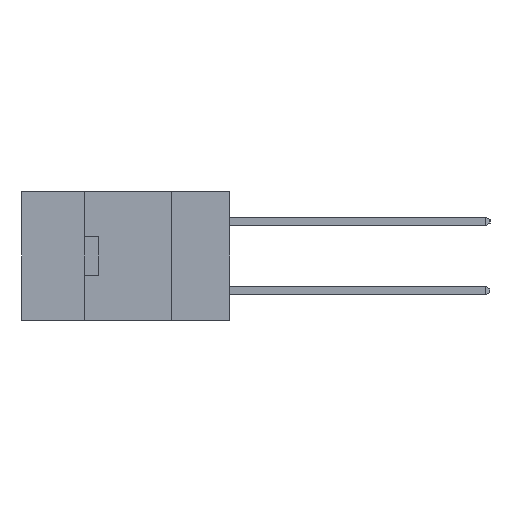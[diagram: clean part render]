
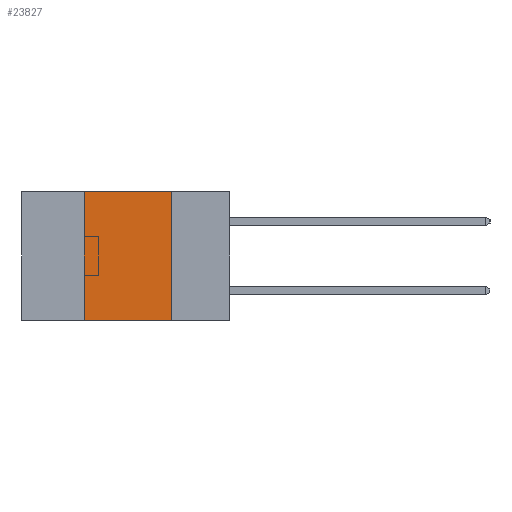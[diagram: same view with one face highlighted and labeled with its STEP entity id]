
A CAD part, left-side view. The second image highlights one B-rep face of the part: STEP entity #23827.
In plain terms, the highlighted planar face has unit normal (-1, 0, 0).
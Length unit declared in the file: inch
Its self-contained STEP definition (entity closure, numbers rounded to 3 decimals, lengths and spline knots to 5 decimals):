
#2149 = DIRECTION ( 'NONE',  ( 0., 0., -1. ) ) ;
#2356 = AXIS2_PLACEMENT_3D ( 'NONE', #26181, #8780, #2149 ) ;
#2430 = VECTOR ( 'NONE', #9022, 39.37008 ) ;
#4492 = ORIENTED_EDGE ( 'NONE', *, *, #21759, .T. ) ;
#4523 = DIRECTION ( 'NONE',  ( 0., -1., 0. ) ) ;
#6205 = VECTOR ( 'NONE', #4523, 39.37008 ) ;
#6902 = LINE ( 'NONE', #8959, #6205 ) ;
#8360 = LINE ( 'NONE', #17566, #2430 ) ;
#8780 = DIRECTION ( 'NONE',  ( 1., 0., 0. ) ) ;
#8959 = CARTESIAN_POINT ( 'NONE',  ( 0., 0.6, -0.37 ) ) ;
#8987 = EDGE_LOOP ( 'NONE', ( #15368, #24232, #27467, #4492 ) ) ;
#9016 = DIRECTION ( 'NONE',  ( 0., 0., -1. ) ) ;
#9022 = DIRECTION ( 'NONE',  ( 0., -1., 0. ) ) ;
#9438 = CARTESIAN_POINT ( 'NONE',  ( 0., 0.42, 0. ) ) ;
#9773 = VERTEX_POINT ( 'NONE', #10660 ) ;
#10660 = CARTESIAN_POINT ( 'NONE',  ( 0., 0.42, -0.37 ) ) ;
#14492 = EDGE_CURVE ( 'NONE', #25694, #23082, #15551, .T. ) ;
#14854 = VECTOR ( 'NONE', #9016, 39.37008 ) ;
#15368 = ORIENTED_EDGE ( 'NONE', *, *, #14492, .F. ) ;
#15551 = LINE ( 'NONE', #21920, #14854 ) ;
#16694 = VERTEX_POINT ( 'NONE', #9438 ) ;
#16980 = CARTESIAN_POINT ( 'NONE',  ( 0., 0.17, -0.37 ) ) ;
#17566 = CARTESIAN_POINT ( 'NONE',  ( 0., 0.6, 0. ) ) ;
#18931 = FACE_OUTER_BOUND ( 'NONE', #8987, .T. ) ;
#19564 = DIRECTION ( 'NONE',  ( 0., 0., 1. ) ) ;
#20289 = EDGE_CURVE ( 'NONE', #16694, #25694, #8360, .T. ) ;
#21759 = EDGE_CURVE ( 'NONE', #9773, #23082, #6902, .T. ) ;
#21834 = VECTOR ( 'NONE', #19564, 39.37008 ) ;
#21920 = CARTESIAN_POINT ( 'NONE',  ( 0., 0.17, -0.37 ) ) ;
#23082 = VERTEX_POINT ( 'NONE', #16980 ) ;
#23827 = ADVANCED_FACE ( 'NONE', ( #18931 ), #28324, .F. ) ;
#24232 = ORIENTED_EDGE ( 'NONE', *, *, #20289, .F. ) ;
#25521 = CARTESIAN_POINT ( 'NONE',  ( 0., 0.17, 0. ) ) ;
#25694 = VERTEX_POINT ( 'NONE', #25521 ) ;
#26166 = EDGE_CURVE ( 'NONE', #9773, #16694, #27631, .T. ) ;
#26181 = CARTESIAN_POINT ( 'NONE',  ( 0., 0.6, 0. ) ) ;
#27467 = ORIENTED_EDGE ( 'NONE', *, *, #26166, .F. ) ;
#27631 = LINE ( 'NONE', #28207, #21834 ) ;
#28207 = CARTESIAN_POINT ( 'NONE',  ( 0., 0.42, -0.37 ) ) ;
#28324 = PLANE ( 'NONE',  #2356 ) ;
